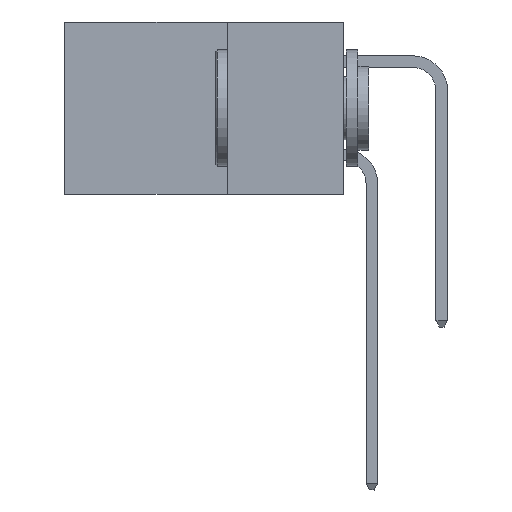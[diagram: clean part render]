
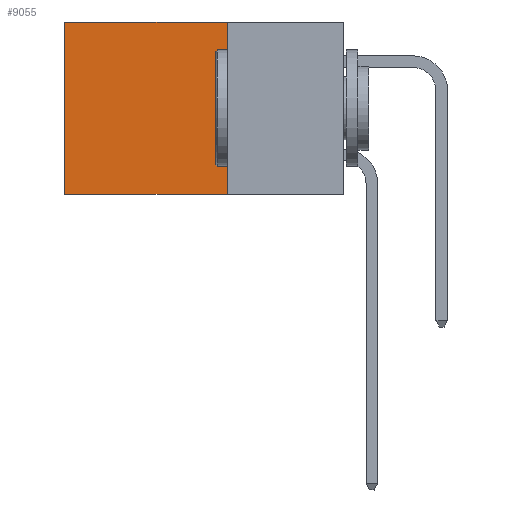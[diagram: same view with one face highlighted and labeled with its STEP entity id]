
A CAD part, left-side view. The second image highlights one B-rep face of the part: STEP entity #9055.
In plain terms, the highlighted planar face has unit normal (-1, 0, 0).
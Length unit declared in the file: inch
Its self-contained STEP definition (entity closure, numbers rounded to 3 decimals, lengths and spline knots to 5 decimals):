
#260 = ORIENTED_EDGE ( 'NONE', *, *, #3682, .F. ) ;
#431 = CARTESIAN_POINT ( 'NONE',  ( 0.298, 0.6, 0. ) ) ;
#875 = EDGE_CURVE ( 'NONE', #10776, #9455, #3747, .T. ) ;
#896 = DIRECTION ( 'NONE',  ( 1., 0., 0. ) ) ;
#1548 = EDGE_CURVE ( 'NONE', #10776, #11400, #6552, .T. ) ;
#1998 = EDGE_CURVE ( 'NONE', #11400, #10860, #10761, .T. ) ;
#2138 = DIRECTION ( 'NONE',  ( 0., 1., 0. ) ) ;
#2205 = LINE ( 'NONE', #3139, #11582 ) ;
#2457 = DIRECTION ( 'NONE',  ( 0., 1., 0. ) ) ;
#3139 = CARTESIAN_POINT ( 'NONE',  ( 0.298, 0.25, -0.37 ) ) ;
#3153 = AXIS2_PLACEMENT_3D ( 'NONE', #3772, #896, #10090 ) ;
#3354 = ORIENTED_EDGE ( 'NONE', *, *, #1998, .T. ) ;
#3682 = EDGE_CURVE ( 'NONE', #9455, #10860, #2205, .T. ) ;
#3747 = LINE ( 'NONE', #9616, #10686 ) ;
#3772 = CARTESIAN_POINT ( 'NONE',  ( 0.298, 0.25, 0. ) ) ;
#4123 = CARTESIAN_POINT ( 'NONE',  ( 0.298, 0.25, 0. ) ) ;
#4146 = VECTOR ( 'NONE', #2457, 39.37008 ) ;
#4340 = FACE_OUTER_BOUND ( 'NONE', #11743, .T. ) ;
#5092 = VECTOR ( 'NONE', #8412, 39.37008 ) ;
#6011 = CARTESIAN_POINT ( 'NONE',  ( 0.298, 0.25, 0. ) ) ;
#6383 = CARTESIAN_POINT ( 'NONE',  ( 0.298, 0.6, 0. ) ) ;
#6552 = LINE ( 'NONE', #6011, #4146 ) ;
#8412 = DIRECTION ( 'NONE',  ( 0., 0., -1. ) ) ;
#8513 = ORIENTED_EDGE ( 'NONE', *, *, #875, .F. ) ;
#8758 = DIRECTION ( 'NONE',  ( 0., 0., -1. ) ) ;
#9055 = ADVANCED_FACE ( 'NONE', ( #4340 ), #9174, .F. ) ;
#9174 = PLANE ( 'NONE',  #3153 ) ;
#9260 = ORIENTED_EDGE ( 'NONE', *, *, #1548, .T. ) ;
#9455 = VERTEX_POINT ( 'NONE', #9643 ) ;
#9616 = CARTESIAN_POINT ( 'NONE',  ( 0.298, 0.25, 0. ) ) ;
#9643 = CARTESIAN_POINT ( 'NONE',  ( 0.298, 0.25, -0.37 ) ) ;
#10090 = DIRECTION ( 'NONE',  ( 0., 0., -1. ) ) ;
#10503 = CARTESIAN_POINT ( 'NONE',  ( 0.298, 0.6, -0.37 ) ) ;
#10686 = VECTOR ( 'NONE', #8758, 39.37008 ) ;
#10761 = LINE ( 'NONE', #431, #5092 ) ;
#10776 = VERTEX_POINT ( 'NONE', #4123 ) ;
#10860 = VERTEX_POINT ( 'NONE', #10503 ) ;
#11400 = VERTEX_POINT ( 'NONE', #6383 ) ;
#11582 = VECTOR ( 'NONE', #2138, 39.37008 ) ;
#11743 = EDGE_LOOP ( 'NONE', ( #3354, #260, #8513, #9260 ) ) ;
